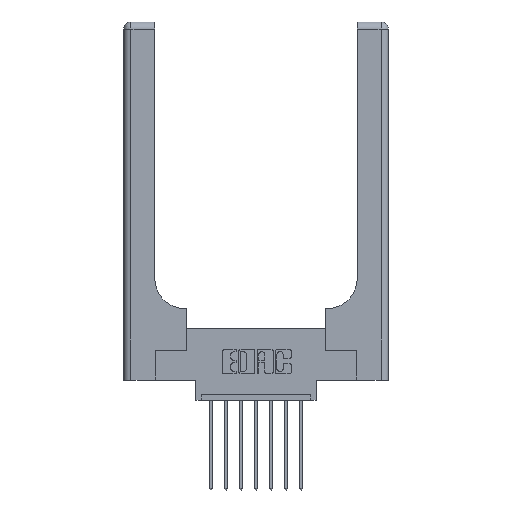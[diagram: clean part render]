
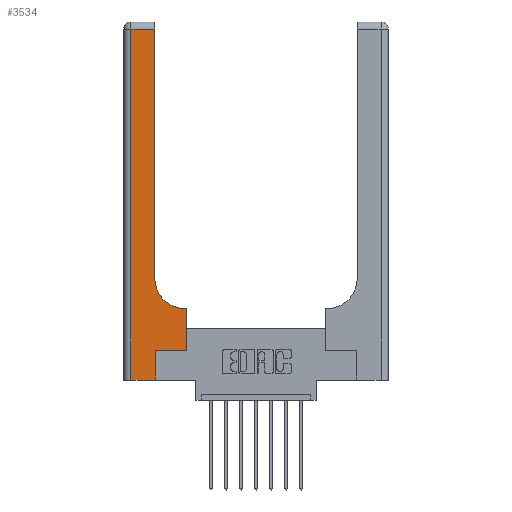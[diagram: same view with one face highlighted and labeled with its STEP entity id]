
A CAD part, top view. The second image highlights one B-rep face of the part: STEP entity #3534.
In plain terms, the highlighted planar face has unit normal (0, 0, 1).
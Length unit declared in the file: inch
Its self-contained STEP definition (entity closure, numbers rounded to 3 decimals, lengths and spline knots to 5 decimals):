
#81 = EDGE_CURVE ( 'NONE', #6773, #4872, #12632, .T. ) ;
#192 = CARTESIAN_POINT ( 'NONE',  ( 0.26, 0.85, 0.37 ) ) ;
#211 = AXIS2_PLACEMENT_3D ( 'NONE', #12738, #13865, #10604 ) ;
#433 = VECTOR ( 'NONE', #12745, 39.37008 ) ;
#500 = LINE ( 'NONE', #9253, #3997 ) ;
#579 = ORIENTED_EDGE ( 'NONE', *, *, #81, .T. ) ;
#695 = CARTESIAN_POINT ( 'NONE',  ( 0.06, 3., 0.37 ) ) ;
#913 = DIRECTION ( 'NONE',  ( 0., 0., -1. ) ) ;
#1377 = VECTOR ( 'NONE', #2781, 39.37008 ) ;
#1801 = DIRECTION ( 'NONE',  ( 1., 0., 0. ) ) ;
#1830 = DIRECTION ( 'NONE',  ( 0., 1., 0. ) ) ;
#2164 = CARTESIAN_POINT ( 'NONE',  ( 0.265, 0.25, 0.37 ) ) ;
#2447 = VECTOR ( 'NONE', #10946, 39.37008 ) ;
#2547 = VECTOR ( 'NONE', #4066, 39.37008 ) ;
#2735 = CARTESIAN_POINT ( 'NONE',  ( 0.265, 0.25, 0.37 ) ) ;
#2781 = DIRECTION ( 'NONE',  ( -1., 0., 0. ) ) ;
#2936 = EDGE_CURVE ( 'NONE', #4621, #3834, #500, .T. ) ;
#3162 = DIRECTION ( 'NONE',  ( 0., 1., 0. ) ) ;
#3534 = ADVANCED_FACE ( 'NONE', ( #12759 ), #14239, .F. ) ;
#3783 = LINE ( 'NONE', #11747, #14345 ) ;
#3804 = EDGE_CURVE ( 'NONE', #3834, #6797, #3783, .T. ) ;
#3834 = VERTEX_POINT ( 'NONE', #7742 ) ;
#3997 = VECTOR ( 'NONE', #1801, 39.37008 ) ;
#4066 = DIRECTION ( 'NONE',  ( 0., -1., 0. ) ) ;
#4084 = ORIENTED_EDGE ( 'NONE', *, *, #5480, .T. ) ;
#4621 = VERTEX_POINT ( 'NONE', #12802 ) ;
#4872 = VERTEX_POINT ( 'NONE', #13967 ) ;
#5095 = EDGE_CURVE ( 'NONE', #4872, #6642, #7621, .T. ) ;
#5466 = ORIENTED_EDGE ( 'NONE', *, *, #6881, .T. ) ;
#5480 = EDGE_CURVE ( 'NONE', #10488, #4621, #9473, .T. ) ;
#5983 = DIRECTION ( 'NONE',  ( 0., 1., 0. ) ) ;
#6642 = VERTEX_POINT ( 'NONE', #192 ) ;
#6660 = LINE ( 'NONE', #13992, #6835 ) ;
#6674 = ORIENTED_EDGE ( 'NONE', *, *, #12226, .T. ) ;
#6773 = VERTEX_POINT ( 'NONE', #8173 ) ;
#6797 = VERTEX_POINT ( 'NONE', #2735 ) ;
#6835 = VECTOR ( 'NONE', #1830, 39.37008 ) ;
#6881 = EDGE_CURVE ( 'NONE', #8582, #10488, #12516, .T. ) ;
#7222 = EDGE_CURVE ( 'NONE', #6642, #8582, #12560, .T. ) ;
#7423 = ORIENTED_EDGE ( 'NONE', *, *, #5095, .T. ) ;
#7449 = CARTESIAN_POINT ( 'NONE',  ( 0.26, 0.6, 0.37 ) ) ;
#7570 = CARTESIAN_POINT ( 'NONE',  ( 0.51, 0.85, 0.37 ) ) ;
#7621 = CIRCLE ( 'NONE', #9678, 0.25 ) ;
#7742 = CARTESIAN_POINT ( 'NONE',  ( 0.265, 0., 0.37 ) ) ;
#7895 = VERTEX_POINT ( 'NONE', #13727 ) ;
#8084 = VECTOR ( 'NONE', #5983, 39.37008 ) ;
#8173 = CARTESIAN_POINT ( 'NONE',  ( 0.528, 0.6, 0.37 ) ) ;
#8195 = ORIENTED_EDGE ( 'NONE', *, *, #7222, .T. ) ;
#8582 = VERTEX_POINT ( 'NONE', #9584 ) ;
#8756 = DIRECTION ( 'NONE',  ( 1., 0., 0. ) ) ;
#9062 = EDGE_LOOP ( 'NONE', ( #8195, #5466, #4084, #12030, #13512, #6674, #14090, #579, #7423 ) ) ;
#9205 = LINE ( 'NONE', #2164, #2447 ) ;
#9253 = CARTESIAN_POINT ( 'NONE',  ( 0., 0., 0.37 ) ) ;
#9473 = LINE ( 'NONE', #695, #2547 ) ;
#9584 = CARTESIAN_POINT ( 'NONE',  ( 0.26, 2.94, 0.37 ) ) ;
#9678 = AXIS2_PLACEMENT_3D ( 'NONE', #7570, #913, #8756 ) ;
#10012 = EDGE_CURVE ( 'NONE', #7895, #6773, #6660, .T. ) ;
#10488 = VERTEX_POINT ( 'NONE', #13651 ) ;
#10604 = DIRECTION ( 'NONE',  ( -1., 0., 0. ) ) ;
#10946 = DIRECTION ( 'NONE',  ( 1., 0., 0. ) ) ;
#11747 = CARTESIAN_POINT ( 'NONE',  ( 0.265, 0., 0.37 ) ) ;
#12030 = ORIENTED_EDGE ( 'NONE', *, *, #2936, .T. ) ;
#12226 = EDGE_CURVE ( 'NONE', #6797, #7895, #9205, .T. ) ;
#12516 = LINE ( 'NONE', #12851, #433 ) ;
#12560 = LINE ( 'NONE', #13560, #8084 ) ;
#12632 = LINE ( 'NONE', #7449, #1377 ) ;
#12738 = CARTESIAN_POINT ( 'NONE',  ( 0., 3., 0.37 ) ) ;
#12745 = DIRECTION ( 'NONE',  ( -1., 0., 0. ) ) ;
#12759 = FACE_OUTER_BOUND ( 'NONE', #9062, .T. ) ;
#12802 = CARTESIAN_POINT ( 'NONE',  ( 0.06, 0., 0.37 ) ) ;
#12851 = CARTESIAN_POINT ( 'NONE',  ( 0., 2.94, 0.37 ) ) ;
#13512 = ORIENTED_EDGE ( 'NONE', *, *, #3804, .T. ) ;
#13560 = CARTESIAN_POINT ( 'NONE',  ( 0.26, 3., 0.37 ) ) ;
#13651 = CARTESIAN_POINT ( 'NONE',  ( 0.06, 2.94, 0.37 ) ) ;
#13727 = CARTESIAN_POINT ( 'NONE',  ( 0.528, 0.25, 0.37 ) ) ;
#13865 = DIRECTION ( 'NONE',  ( 0., 0., -1. ) ) ;
#13967 = CARTESIAN_POINT ( 'NONE',  ( 0.51, 0.6, 0.37 ) ) ;
#13992 = CARTESIAN_POINT ( 'NONE',  ( 0.528, 0.25, 0.37 ) ) ;
#14090 = ORIENTED_EDGE ( 'NONE', *, *, #10012, .T. ) ;
#14239 = PLANE ( 'NONE',  #211 ) ;
#14345 = VECTOR ( 'NONE', #3162, 39.37008 ) ;
